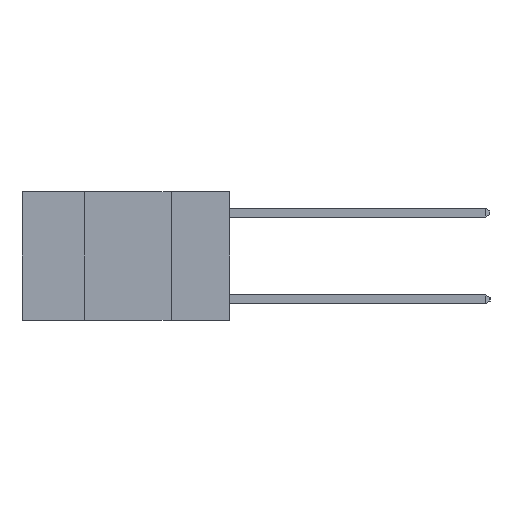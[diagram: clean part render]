
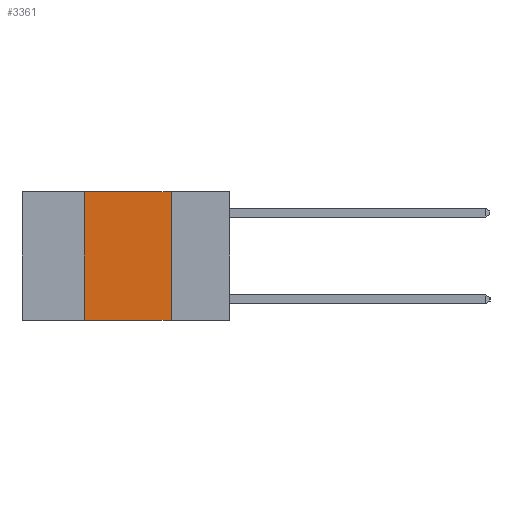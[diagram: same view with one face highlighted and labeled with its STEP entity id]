
A CAD part, left-side view. The second image highlights one B-rep face of the part: STEP entity #3361.
In plain terms, the highlighted planar face has unit normal (-1, 0, 0).
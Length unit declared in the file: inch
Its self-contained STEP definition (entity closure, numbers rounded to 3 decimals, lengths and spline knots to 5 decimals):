
#193 = EDGE_CURVE ( 'NONE', #7394, #8628, #4370, .T. ) ;
#217 = CARTESIAN_POINT ( 'NONE',  ( 0., 0.42, 0. ) ) ;
#279 = VECTOR ( 'NONE', #1127, 39.37008 ) ;
#427 = CARTESIAN_POINT ( 'NONE',  ( 0., 0.6, 0. ) ) ;
#853 = CARTESIAN_POINT ( 'NONE',  ( 0., 0.6, -0.37 ) ) ;
#1127 = DIRECTION ( 'NONE',  ( 0., -1., 0. ) ) ;
#1435 = EDGE_CURVE ( 'NONE', #7603, #2312, #2119, .T. ) ;
#1836 = DIRECTION ( 'NONE',  ( 0., 0., -1. ) ) ;
#1921 = CARTESIAN_POINT ( 'NONE',  ( 0., 0.17, 0. ) ) ;
#2119 = LINE ( 'NONE', #853, #279 ) ;
#2312 = VERTEX_POINT ( 'NONE', #7401 ) ;
#2604 = VECTOR ( 'NONE', #3702, 39.37008 ) ;
#2645 = EDGE_CURVE ( 'NONE', #8628, #2312, #7583, .T. ) ;
#3075 = ORIENTED_EDGE ( 'NONE', *, *, #7257, .F. ) ;
#3288 = CARTESIAN_POINT ( 'NONE',  ( 0., 0.42, -0.37 ) ) ;
#3361 = ADVANCED_FACE ( 'NONE', ( #4268 ), #5158, .F. ) ;
#3702 = DIRECTION ( 'NONE',  ( 0., -1., 0. ) ) ;
#3895 = ORIENTED_EDGE ( 'NONE', *, *, #1435, .T. ) ;
#3912 = ORIENTED_EDGE ( 'NONE', *, *, #2645, .F. ) ;
#4124 = CARTESIAN_POINT ( 'NONE',  ( 0., 0.42, 0. ) ) ;
#4268 = FACE_OUTER_BOUND ( 'NONE', #5168, .T. ) ;
#4370 = LINE ( 'NONE', #7545, #2604 ) ;
#4939 = VECTOR ( 'NONE', #7542, 39.37008 ) ;
#5059 = AXIS2_PLACEMENT_3D ( 'NONE', #427, #5885, #1836 ) ;
#5158 = PLANE ( 'NONE',  #5059 ) ;
#5168 = EDGE_LOOP ( 'NONE', ( #3912, #7616, #3075, #3895 ) ) ;
#5803 = CARTESIAN_POINT ( 'NONE',  ( 0., 0.17, 0. ) ) ;
#5815 = VECTOR ( 'NONE', #7825, 39.37008 ) ;
#5885 = DIRECTION ( 'NONE',  ( 1., 0., 0. ) ) ;
#6754 = LINE ( 'NONE', #4124, #4939 ) ;
#7257 = EDGE_CURVE ( 'NONE', #7603, #7394, #6754, .T. ) ;
#7394 = VERTEX_POINT ( 'NONE', #217 ) ;
#7401 = CARTESIAN_POINT ( 'NONE',  ( 0., 0.17, -0.37 ) ) ;
#7542 = DIRECTION ( 'NONE',  ( 0., 0., 1. ) ) ;
#7545 = CARTESIAN_POINT ( 'NONE',  ( 0., 0.6, 0. ) ) ;
#7583 = LINE ( 'NONE', #5803, #5815 ) ;
#7603 = VERTEX_POINT ( 'NONE', #3288 ) ;
#7616 = ORIENTED_EDGE ( 'NONE', *, *, #193, .F. ) ;
#7825 = DIRECTION ( 'NONE',  ( 0., 0., -1. ) ) ;
#8628 = VERTEX_POINT ( 'NONE', #1921 ) ;
